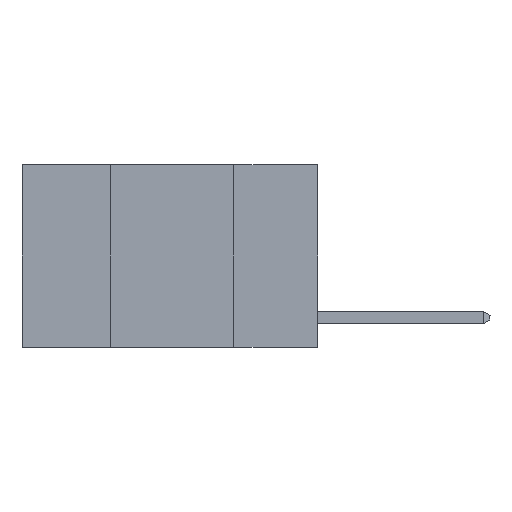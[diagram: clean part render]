
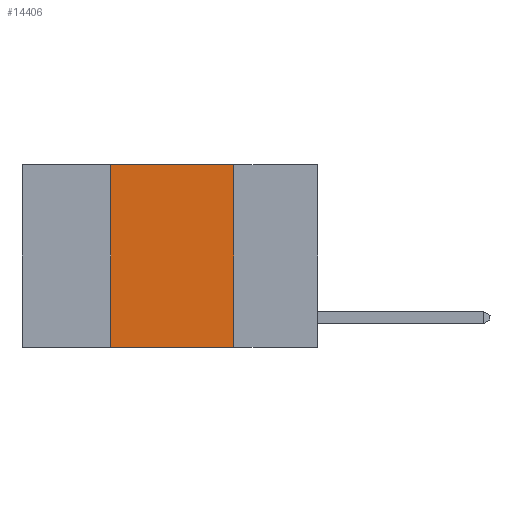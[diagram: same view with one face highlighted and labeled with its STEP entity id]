
A CAD part, left-side view. The second image highlights one B-rep face of the part: STEP entity #14406.
In plain terms, the highlighted planar face has unit normal (-1, 0, 0).
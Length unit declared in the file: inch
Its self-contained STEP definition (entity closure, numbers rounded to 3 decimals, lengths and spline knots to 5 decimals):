
#249 = CARTESIAN_POINT ( 'NONE',  ( 0., 0.42, 0. ) ) ;
#319 = CARTESIAN_POINT ( 'NONE',  ( 0., 0.6, 0. ) ) ;
#1175 = DIRECTION ( 'NONE',  ( 0., -1., 0. ) ) ;
#1316 = CARTESIAN_POINT ( 'NONE',  ( 0., 0.42, 0. ) ) ;
#2518 = VECTOR ( 'NONE', #10725, 39.37008 ) ;
#2930 = LINE ( 'NONE', #16711, #18721 ) ;
#3323 = VERTEX_POINT ( 'NONE', #11957 ) ;
#3604 = LINE ( 'NONE', #12869, #17449 ) ;
#3965 = ORIENTED_EDGE ( 'NONE', *, *, #8407, .F. ) ;
#4454 = CARTESIAN_POINT ( 'NONE',  ( 0., 0.6, -0.37 ) ) ;
#5025 = PLANE ( 'NONE',  #5342 ) ;
#5056 = EDGE_LOOP ( 'NONE', ( #16594, #3965, #14773, #5127 ) ) ;
#5127 = ORIENTED_EDGE ( 'NONE', *, *, #6070, .T. ) ;
#5342 = AXIS2_PLACEMENT_3D ( 'NONE', #319, #18824, #17579 ) ;
#6070 = EDGE_CURVE ( 'NONE', #7071, #3323, #7629, .T. ) ;
#6343 = VERTEX_POINT ( 'NONE', #1316 ) ;
#7071 = VERTEX_POINT ( 'NONE', #9811 ) ;
#7629 = LINE ( 'NONE', #4454, #2518 ) ;
#8407 = EDGE_CURVE ( 'NONE', #6343, #17136, #2930, .T. ) ;
#9089 = EDGE_CURVE ( 'NONE', #17136, #3323, #3604, .T. ) ;
#9811 = CARTESIAN_POINT ( 'NONE',  ( 0., 0.42, -0.37 ) ) ;
#10307 = VECTOR ( 'NONE', #12783, 39.37008 ) ;
#10725 = DIRECTION ( 'NONE',  ( 0., -1., 0. ) ) ;
#11957 = CARTESIAN_POINT ( 'NONE',  ( 0., 0.17, -0.37 ) ) ;
#12686 = LINE ( 'NONE', #249, #10307 ) ;
#12783 = DIRECTION ( 'NONE',  ( 0., 0., 1. ) ) ;
#12869 = CARTESIAN_POINT ( 'NONE',  ( 0., 0.17, 0. ) ) ;
#14406 = ADVANCED_FACE ( 'NONE', ( #18932 ), #5025, .F. ) ;
#14519 = DIRECTION ( 'NONE',  ( 0., 0., -1. ) ) ;
#14773 = ORIENTED_EDGE ( 'NONE', *, *, #19733, .F. ) ;
#16594 = ORIENTED_EDGE ( 'NONE', *, *, #9089, .F. ) ;
#16711 = CARTESIAN_POINT ( 'NONE',  ( 0., 0.6, 0. ) ) ;
#16776 = CARTESIAN_POINT ( 'NONE',  ( 0., 0.17, 0. ) ) ;
#17136 = VERTEX_POINT ( 'NONE', #16776 ) ;
#17449 = VECTOR ( 'NONE', #14519, 39.37008 ) ;
#17579 = DIRECTION ( 'NONE',  ( 0., 0., -1. ) ) ;
#18721 = VECTOR ( 'NONE', #1175, 39.37008 ) ;
#18824 = DIRECTION ( 'NONE',  ( 1., 0., 0. ) ) ;
#18932 = FACE_OUTER_BOUND ( 'NONE', #5056, .T. ) ;
#19733 = EDGE_CURVE ( 'NONE', #7071, #6343, #12686, .T. ) ;
